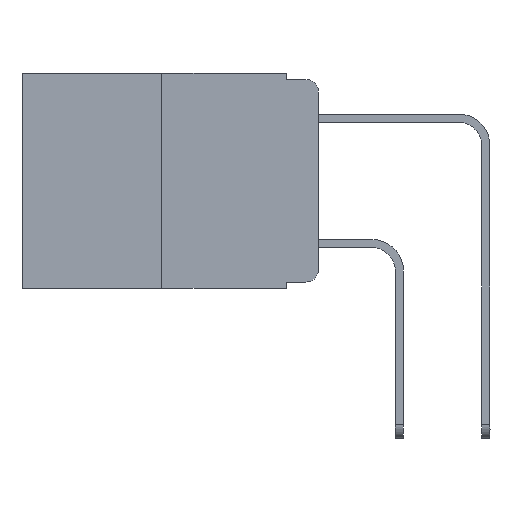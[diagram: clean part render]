
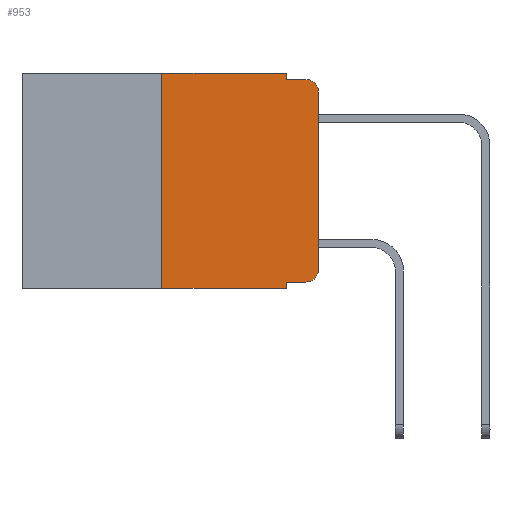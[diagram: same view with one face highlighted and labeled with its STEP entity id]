
A CAD part, left-side view. The second image highlights one B-rep face of the part: STEP entity #953.
In plain terms, the highlighted planar face has unit normal (-1, 0, 0).
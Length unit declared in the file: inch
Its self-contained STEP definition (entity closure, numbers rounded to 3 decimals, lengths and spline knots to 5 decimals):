
#180 = LINE ( 'NONE', #6817, #12372 ) ;
#326 = CARTESIAN_POINT ( 'NONE',  ( 0., 0.02, -0.03 ) ) ;
#578 = CARTESIAN_POINT ( 'NONE',  ( 0., 0.25, 0. ) ) ;
#953 = ADVANCED_FACE ( 'NONE', ( #7081 ), #10933, .F. ) ;
#1408 = ORIENTED_EDGE ( 'NONE', *, *, #16900, .F. ) ;
#1542 = LINE ( 'NONE', #13492, #11521 ) ;
#1731 = CARTESIAN_POINT ( 'NONE',  ( 0., 0.051, -0.01 ) ) ;
#1823 = CARTESIAN_POINT ( 'NONE',  ( 0., 0.051, -0.333 ) ) ;
#2528 = LINE ( 'NONE', #3652, #6754 ) ;
#3039 = AXIS2_PLACEMENT_3D ( 'NONE', #326, #16066, #4279 ) ;
#3175 = CARTESIAN_POINT ( 'NONE',  ( 0., 0.051, 0. ) ) ;
#3394 = CARTESIAN_POINT ( 'NONE',  ( 0., 0., -0.313 ) ) ;
#3445 = AXIS2_PLACEMENT_3D ( 'NONE', #7597, #10341, #11456 ) ;
#3632 = ORIENTED_EDGE ( 'NONE', *, *, #4467, .T. ) ;
#3652 = CARTESIAN_POINT ( 'NONE',  ( 0., 0.051, -0.01 ) ) ;
#3854 = ORIENTED_EDGE ( 'NONE', *, *, #11391, .F. ) ;
#3867 = CIRCLE ( 'NONE', #3039, 0.02 ) ;
#4279 = DIRECTION ( 'NONE',  ( 0., 0., -1. ) ) ;
#4299 = VERTEX_POINT ( 'NONE', #8489 ) ;
#4406 = EDGE_LOOP ( 'NONE', ( #13867, #12055, #13947, #1408, #3854, #6995, #10478, #10839, #3632, #5699 ) ) ;
#4414 = DIRECTION ( 'NONE',  ( 1., 0., 0. ) ) ;
#4467 = EDGE_CURVE ( 'NONE', #15398, #14994, #10196, .T. ) ;
#4549 = CIRCLE ( 'NONE', #3445, 0.02 ) ;
#4761 = DIRECTION ( 'NONE',  ( 0., 0., 1. ) ) ;
#4767 = VERTEX_POINT ( 'NONE', #578 ) ;
#4816 = VERTEX_POINT ( 'NONE', #8965 ) ;
#5062 = CARTESIAN_POINT ( 'NONE',  ( 0., 0.051, -0.333 ) ) ;
#5084 = VERTEX_POINT ( 'NONE', #3394 ) ;
#5325 = DIRECTION ( 'NONE',  ( 0., -1., 0. ) ) ;
#5542 = VERTEX_POINT ( 'NONE', #15064 ) ;
#5699 = ORIENTED_EDGE ( 'NONE', *, *, #8625, .T. ) ;
#6754 = VECTOR ( 'NONE', #12754, 39.37008 ) ;
#6817 = CARTESIAN_POINT ( 'NONE',  ( 0., 0.051, 0. ) ) ;
#6834 = EDGE_CURVE ( 'NONE', #4816, #4299, #12300, .T. ) ;
#6995 = ORIENTED_EDGE ( 'NONE', *, *, #12053, .F. ) ;
#6998 = CARTESIAN_POINT ( 'NONE',  ( 0., 0.473, -0.343 ) ) ;
#7081 = FACE_OUTER_BOUND ( 'NONE', #4406, .T. ) ;
#7597 = CARTESIAN_POINT ( 'NONE',  ( 0., 0.02, -0.313 ) ) ;
#7626 = CARTESIAN_POINT ( 'NONE',  ( 0., 0., -0.03 ) ) ;
#8489 = CARTESIAN_POINT ( 'NONE',  ( 0., 0.051, -0.343 ) ) ;
#8625 = EDGE_CURVE ( 'NONE', #14994, #5084, #4549, .T. ) ;
#8647 = EDGE_CURVE ( 'NONE', #10561, #5542, #2528, .T. ) ;
#8965 = CARTESIAN_POINT ( 'NONE',  ( 0., 0.25, -0.343 ) ) ;
#9342 = CARTESIAN_POINT ( 'NONE',  ( 0., 0.473, 0. ) ) ;
#9425 = VECTOR ( 'NONE', #13132, 39.37008 ) ;
#9475 = EDGE_CURVE ( 'NONE', #15398, #4299, #11338, .T. ) ;
#9522 = DIRECTION ( 'NONE',  ( 0., 0., 1. ) ) ;
#9798 = VECTOR ( 'NONE', #11595, 39.37008 ) ;
#9860 = AXIS2_PLACEMENT_3D ( 'NONE', #12478, #4414, #13606 ) ;
#9989 = LINE ( 'NONE', #16706, #12026 ) ;
#10196 = LINE ( 'NONE', #5062, #9425 ) ;
#10341 = DIRECTION ( 'NONE',  ( -1., 0., 0. ) ) ;
#10386 = CARTESIAN_POINT ( 'NONE',  ( 0., 0.051, 0. ) ) ;
#10478 = ORIENTED_EDGE ( 'NONE', *, *, #6834, .T. ) ;
#10561 = VERTEX_POINT ( 'NONE', #1731 ) ;
#10839 = ORIENTED_EDGE ( 'NONE', *, *, #9475, .F. ) ;
#10933 = PLANE ( 'NONE',  #9860 ) ;
#11338 = LINE ( 'NONE', #10386, #9798 ) ;
#11391 = EDGE_CURVE ( 'NONE', #4767, #14025, #13221, .T. ) ;
#11456 = DIRECTION ( 'NONE',  ( 0., 0., -1. ) ) ;
#11521 = VECTOR ( 'NONE', #9522, 39.37008 ) ;
#11595 = DIRECTION ( 'NONE',  ( 0., 0., -1. ) ) ;
#12026 = VECTOR ( 'NONE', #4761, 39.37008 ) ;
#12053 = EDGE_CURVE ( 'NONE', #4816, #4767, #9989, .T. ) ;
#12055 = ORIENTED_EDGE ( 'NONE', *, *, #14455, .T. ) ;
#12273 = VECTOR ( 'NONE', #5325, 39.37008 ) ;
#12300 = LINE ( 'NONE', #6998, #16515 ) ;
#12372 = VECTOR ( 'NONE', #16100, 39.37008 ) ;
#12417 = CARTESIAN_POINT ( 'NONE',  ( 0., 0.02, -0.333 ) ) ;
#12478 = CARTESIAN_POINT ( 'NONE',  ( 0., 0.473, 0. ) ) ;
#12754 = DIRECTION ( 'NONE',  ( 0., -1., 0. ) ) ;
#13132 = DIRECTION ( 'NONE',  ( 0., -1., 0. ) ) ;
#13221 = LINE ( 'NONE', #9342, #12273 ) ;
#13492 = CARTESIAN_POINT ( 'NONE',  ( 0., 0., 0. ) ) ;
#13606 = DIRECTION ( 'NONE',  ( 0., 0., -1. ) ) ;
#13867 = ORIENTED_EDGE ( 'NONE', *, *, #13911, .T. ) ;
#13911 = EDGE_CURVE ( 'NONE', #5084, #14237, #1542, .T. ) ;
#13947 = ORIENTED_EDGE ( 'NONE', *, *, #8647, .F. ) ;
#14025 = VERTEX_POINT ( 'NONE', #3175 ) ;
#14237 = VERTEX_POINT ( 'NONE', #7626 ) ;
#14455 = EDGE_CURVE ( 'NONE', #14237, #5542, #3867, .T. ) ;
#14994 = VERTEX_POINT ( 'NONE', #12417 ) ;
#15064 = CARTESIAN_POINT ( 'NONE',  ( 0., 0.02, -0.01 ) ) ;
#15243 = DIRECTION ( 'NONE',  ( 0., -1., 0. ) ) ;
#15398 = VERTEX_POINT ( 'NONE', #1823 ) ;
#16066 = DIRECTION ( 'NONE',  ( -1., 0., 0. ) ) ;
#16100 = DIRECTION ( 'NONE',  ( 0., 0., -1. ) ) ;
#16515 = VECTOR ( 'NONE', #15243, 39.37008 ) ;
#16706 = CARTESIAN_POINT ( 'NONE',  ( 0., 0.25, 0. ) ) ;
#16900 = EDGE_CURVE ( 'NONE', #14025, #10561, #180, .T. ) ;
